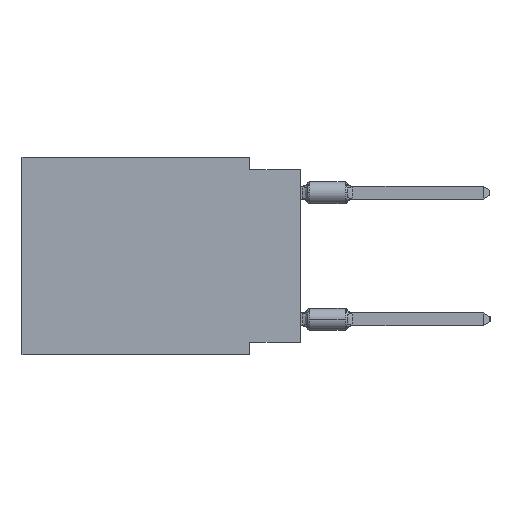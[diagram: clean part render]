
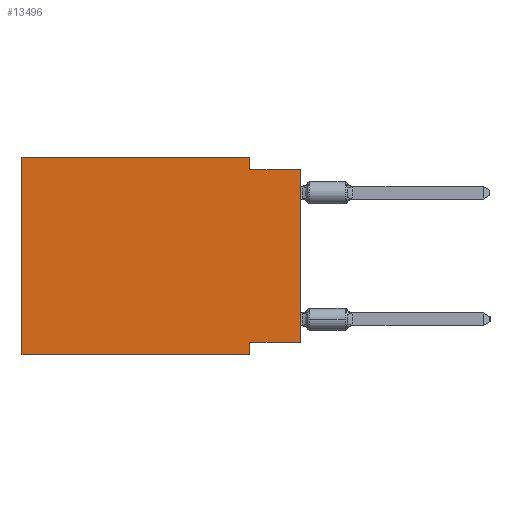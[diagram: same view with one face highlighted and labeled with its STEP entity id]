
A CAD part, left-side view. The second image highlights one B-rep face of the part: STEP entity #13496.
In plain terms, the highlighted planar face has unit normal (-1, 0, 0).
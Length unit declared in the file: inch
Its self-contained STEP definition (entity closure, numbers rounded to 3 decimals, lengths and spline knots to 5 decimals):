
#744 = VECTOR ( 'NONE', #21392, 39.37008 ) ;
#968 = VERTEX_POINT ( 'NONE', #1279 ) ;
#1003 = EDGE_CURVE ( 'NONE', #36654, #24496, #21394, .T. ) ;
#1279 = CARTESIAN_POINT ( 'NONE',  ( 0., 0.1, 0. ) ) ;
#1359 = VERTEX_POINT ( 'NONE', #31913 ) ;
#1759 = DIRECTION ( 'NONE',  ( 0., 0., -1. ) ) ;
#3304 = VECTOR ( 'NONE', #51388, 39.37008 ) ;
#3616 = LINE ( 'NONE', #39295, #3631 ) ;
#3631 = VECTOR ( 'NONE', #51601, 39.37008 ) ;
#5015 = DIRECTION ( 'NONE',  ( 0., -1., 0. ) ) ;
#6170 = ORIENTED_EDGE ( 'NONE', *, *, #46265, .F. ) ;
#8379 = ORIENTED_EDGE ( 'NONE', *, *, #15928, .T. ) ;
#13496 = ADVANCED_FACE ( 'NONE', ( #39566 ), #27280, .F. ) ;
#15206 = CARTESIAN_POINT ( 'NONE',  ( 0., 0.1, -0.39 ) ) ;
#15928 = EDGE_CURVE ( 'NONE', #36654, #1359, #20074, .T. ) ;
#16241 = VERTEX_POINT ( 'NONE', #36714 ) ;
#17318 = LINE ( 'NONE', #26978, #25126 ) ;
#18145 = EDGE_CURVE ( 'NONE', #50023, #1359, #43052, .T. ) ;
#18432 = VECTOR ( 'NONE', #37434, 39.37008 ) ;
#19312 = LINE ( 'NONE', #37154, #18432 ) ;
#20074 = LINE ( 'NONE', #28289, #3304 ) ;
#20159 = LINE ( 'NONE', #15206, #21302 ) ;
#20230 = DIRECTION ( 'NONE',  ( 0., 1., 0. ) ) ;
#21299 = CARTESIAN_POINT ( 'NONE',  ( 0., 0.1, -0.39 ) ) ;
#21302 = VECTOR ( 'NONE', #1759, 39.37008 ) ;
#21392 = DIRECTION ( 'NONE',  ( 0., -1., 0. ) ) ;
#21394 = LINE ( 'NONE', #46878, #36750 ) ;
#21437 = EDGE_CURVE ( 'NONE', #16241, #49232, #3616, .T. ) ;
#21722 = DIRECTION ( 'NONE',  ( 0., 0., -1. ) ) ;
#21757 = CARTESIAN_POINT ( 'NONE',  ( 0., 0.1, -0.365 ) ) ;
#24496 = VERTEX_POINT ( 'NONE', #21757 ) ;
#25126 = VECTOR ( 'NONE', #30784, 39.37008 ) ;
#25173 = EDGE_CURVE ( 'NONE', #24496, #49232, #20159, .T. ) ;
#26978 = CARTESIAN_POINT ( 'NONE',  ( 0., 0.1, 0. ) ) ;
#27280 = PLANE ( 'NONE',  #43440 ) ;
#28289 = CARTESIAN_POINT ( 'NONE',  ( 0., 0., 0. ) ) ;
#30784 = DIRECTION ( 'NONE',  ( 0., 0., -1. ) ) ;
#31366 = CARTESIAN_POINT ( 'NONE',  ( 0., 0.55, 0. ) ) ;
#31913 = CARTESIAN_POINT ( 'NONE',  ( 0., 0., -0.025 ) ) ;
#33754 = VECTOR ( 'NONE', #5015, 39.37008 ) ;
#33985 = CARTESIAN_POINT ( 'NONE',  ( 0., 0., -0.025 ) ) ;
#34041 = CARTESIAN_POINT ( 'NONE',  ( 0., 0.1, -0.025 ) ) ;
#36654 = VERTEX_POINT ( 'NONE', #44604 ) ;
#36714 = CARTESIAN_POINT ( 'NONE',  ( 0., 0.55, -0.39 ) ) ;
#36750 = VECTOR ( 'NONE', #20230, 39.37008 ) ;
#36851 = CARTESIAN_POINT ( 'NONE',  ( 0., 0.55, 0. ) ) ;
#37154 = CARTESIAN_POINT ( 'NONE',  ( 0., 0.55, 0. ) ) ;
#37222 = EDGE_CURVE ( 'NONE', #16241, #45274, #19312, .T. ) ;
#37434 = DIRECTION ( 'NONE',  ( 0., 0., 1. ) ) ;
#39295 = CARTESIAN_POINT ( 'NONE',  ( 0., 0.55, -0.39 ) ) ;
#39323 = ORIENTED_EDGE ( 'NONE', *, *, #1003, .F. ) ;
#39566 = FACE_OUTER_BOUND ( 'NONE', #45322, .T. ) ;
#39884 = ORIENTED_EDGE ( 'NONE', *, *, #51800, .F. ) ;
#41238 = LINE ( 'NONE', #36851, #33754 ) ;
#43052 = LINE ( 'NONE', #33985, #744 ) ;
#43440 = AXIS2_PLACEMENT_3D ( 'NONE', #31366, #44564, #21722 ) ;
#43604 = ORIENTED_EDGE ( 'NONE', *, *, #25173, .F. ) ;
#43750 = ORIENTED_EDGE ( 'NONE', *, *, #21437, .T. ) ;
#44564 = DIRECTION ( 'NONE',  ( 1., 0., 0. ) ) ;
#44604 = CARTESIAN_POINT ( 'NONE',  ( 0., 0., -0.365 ) ) ;
#45274 = VERTEX_POINT ( 'NONE', #47938 ) ;
#45322 = EDGE_LOOP ( 'NONE', ( #8379, #57646, #39884, #6170, #54260, #43750, #43604, #39323 ) ) ;
#46265 = EDGE_CURVE ( 'NONE', #45274, #968, #41238, .T. ) ;
#46878 = CARTESIAN_POINT ( 'NONE',  ( 0., 0., -0.365 ) ) ;
#47938 = CARTESIAN_POINT ( 'NONE',  ( 0., 0.55, 0. ) ) ;
#49232 = VERTEX_POINT ( 'NONE', #21299 ) ;
#50023 = VERTEX_POINT ( 'NONE', #34041 ) ;
#51388 = DIRECTION ( 'NONE',  ( 0., 0., 1. ) ) ;
#51601 = DIRECTION ( 'NONE',  ( 0., -1., 0. ) ) ;
#51800 = EDGE_CURVE ( 'NONE', #968, #50023, #17318, .T. ) ;
#54260 = ORIENTED_EDGE ( 'NONE', *, *, #37222, .F. ) ;
#57646 = ORIENTED_EDGE ( 'NONE', *, *, #18145, .F. ) ;
